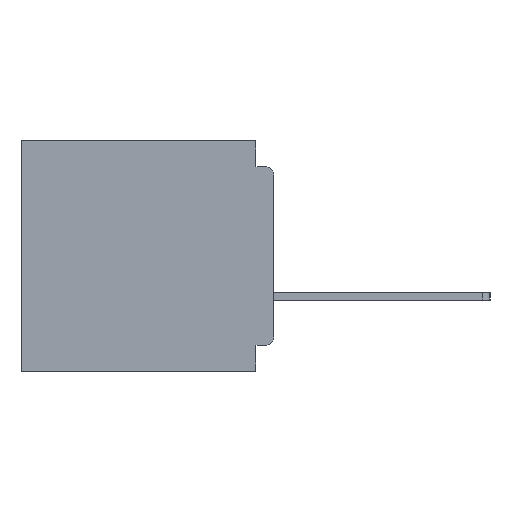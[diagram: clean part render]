
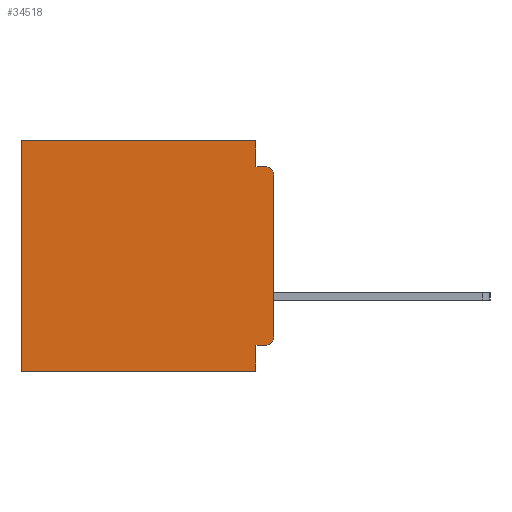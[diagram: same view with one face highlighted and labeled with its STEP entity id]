
A CAD part, left-side view. The second image highlights one B-rep face of the part: STEP entity #34518.
In plain terms, the highlighted planar face has unit normal (-1, 0, 0).
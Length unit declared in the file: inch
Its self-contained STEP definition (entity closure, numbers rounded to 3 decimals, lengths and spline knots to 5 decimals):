
#364 = DIRECTION ( 'NONE',  ( 0., 0., -1. ) ) ;
#880 = VERTEX_POINT ( 'NONE', #19488 ) ;
#1233 = EDGE_CURVE ( 'NONE', #1501, #36022, #8729, .T. ) ;
#1242 = EDGE_CURVE ( 'NONE', #15612, #1501, #24588, .T. ) ;
#1501 = VERTEX_POINT ( 'NONE', #20663 ) ;
#2555 = DIRECTION ( 'NONE',  ( 0., -1., 0. ) ) ;
#2652 = DIRECTION ( 'NONE',  ( -1., 0., 0. ) ) ;
#3565 = VECTOR ( 'NONE', #2555, 39.37008 ) ;
#4012 = LINE ( 'NONE', #10964, #20931 ) ;
#4858 = EDGE_CURVE ( 'NONE', #30091, #30769, #34595, .T. ) ;
#5590 = EDGE_CURVE ( 'NONE', #15612, #20158, #31104, .T. ) ;
#5724 = AXIS2_PLACEMENT_3D ( 'NONE', #21704, #2652, #24870 ) ;
#6927 = CARTESIAN_POINT ( 'NONE',  ( 0.3, 0., -0.4 ) ) ;
#7336 = LINE ( 'NONE', #33890, #24201 ) ;
#7549 = CARTESIAN_POINT ( 'NONE',  ( 0.3, 0., -0.4 ) ) ;
#8361 = ORIENTED_EDGE ( 'NONE', *, *, #8889, .F. ) ;
#8549 = DIRECTION ( 'NONE',  ( -1., 0., 0. ) ) ;
#8682 = AXIS2_PLACEMENT_3D ( 'NONE', #7549, #17140, #39043 ) ;
#8729 = LINE ( 'NONE', #22345, #25586 ) ;
#8889 = EDGE_CURVE ( 'NONE', #20158, #17892, #27850, .T. ) ;
#9455 = VECTOR ( 'NONE', #16141, 39.37008 ) ;
#10663 = VECTOR ( 'NONE', #364, 39.37008 ) ;
#10964 = CARTESIAN_POINT ( 'NONE',  ( 0.3, 0., -0.4 ) ) ;
#12953 = CARTESIAN_POINT ( 'NONE',  ( 0.3, 0.031, -0.4 ) ) ;
#13448 = CARTESIAN_POINT ( 'NONE',  ( 0.3, 0.031, 0. ) ) ;
#13936 = PLANE ( 'NONE',  #8682 ) ;
#14326 = ORIENTED_EDGE ( 'NONE', *, *, #34737, .T. ) ;
#14331 = VECTOR ( 'NONE', #19848, 39.37008 ) ;
#15174 = VECTOR ( 'NONE', #21255, 39.37008 ) ;
#15340 = CARTESIAN_POINT ( 'NONE',  ( 0.3, 0., -0.045 ) ) ;
#15386 = ORIENTED_EDGE ( 'NONE', *, *, #24315, .F. ) ;
#15612 = VERTEX_POINT ( 'NONE', #32898 ) ;
#16141 = DIRECTION ( 'NONE',  ( 0., 0., -1. ) ) ;
#16449 = ORIENTED_EDGE ( 'NONE', *, *, #1233, .T. ) ;
#17140 = DIRECTION ( 'NONE',  ( 1., 0., 0. ) ) ;
#17245 = CARTESIAN_POINT ( 'NONE',  ( 0.3, 0.015, -0.355 ) ) ;
#17627 = CARTESIAN_POINT ( 'NONE',  ( 0.3, 0.031, -0.045 ) ) ;
#17892 = VERTEX_POINT ( 'NONE', #24485 ) ;
#19488 = CARTESIAN_POINT ( 'NONE',  ( 0.3, 0., -0.34 ) ) ;
#19553 = ORIENTED_EDGE ( 'NONE', *, *, #5590, .F. ) ;
#19848 = DIRECTION ( 'NONE',  ( 0., 0., -1. ) ) ;
#20103 = EDGE_CURVE ( 'NONE', #30769, #36022, #4012, .T. ) ;
#20126 = LINE ( 'NONE', #6927, #10663 ) ;
#20158 = VERTEX_POINT ( 'NONE', #17627 ) ;
#20663 = CARTESIAN_POINT ( 'NONE',  ( 0.3, 0.437, 0. ) ) ;
#20697 = CIRCLE ( 'NONE', #5724, 0.015 ) ;
#20931 = VECTOR ( 'NONE', #29861, 39.37008 ) ;
#21123 = DIRECTION ( 'NONE',  ( 0., 0., -1. ) ) ;
#21216 = FACE_OUTER_BOUND ( 'NONE', #29043, .T. ) ;
#21255 = DIRECTION ( 'NONE',  ( 0., 1., 0. ) ) ;
#21395 = CARTESIAN_POINT ( 'NONE',  ( 0.3, 0., 0. ) ) ;
#21704 = CARTESIAN_POINT ( 'NONE',  ( 0.3, 0.015, -0.06 ) ) ;
#22178 = CARTESIAN_POINT ( 'NONE',  ( 0.3, 0.437, -0.4 ) ) ;
#22345 = CARTESIAN_POINT ( 'NONE',  ( 0.3, 0.437, -0.4 ) ) ;
#23362 = EDGE_CURVE ( 'NONE', #25110, #880, #28987, .T. ) ;
#24201 = VECTOR ( 'NONE', #36997, 39.37008 ) ;
#24315 = EDGE_CURVE ( 'NONE', #33473, #880, #20126, .T. ) ;
#24485 = CARTESIAN_POINT ( 'NONE',  ( 0.3, 0.015, -0.045 ) ) ;
#24588 = LINE ( 'NONE', #21395, #15174 ) ;
#24870 = DIRECTION ( 'NONE',  ( 0., 0., -1. ) ) ;
#24985 = CARTESIAN_POINT ( 'NONE',  ( 0.3, 0.031, -0.355 ) ) ;
#25110 = VERTEX_POINT ( 'NONE', #17245 ) ;
#25551 = ORIENTED_EDGE ( 'NONE', *, *, #20103, .F. ) ;
#25586 = VECTOR ( 'NONE', #21123, 39.37008 ) ;
#26497 = EDGE_CURVE ( 'NONE', #25110, #30091, #7336, .T. ) ;
#26961 = AXIS2_PLACEMENT_3D ( 'NONE', #27501, #8549, #30621 ) ;
#27440 = CARTESIAN_POINT ( 'NONE',  ( 0.3, 0., -0.06 ) ) ;
#27501 = CARTESIAN_POINT ( 'NONE',  ( 0.3, 0.015, -0.34 ) ) ;
#27850 = LINE ( 'NONE', #15340, #3565 ) ;
#28987 = CIRCLE ( 'NONE', #26961, 0.015 ) ;
#29043 = EDGE_LOOP ( 'NONE', ( #15386, #14326, #8361, #19553, #30883, #16449, #25551, #31829, #31611, #35173 ) ) ;
#29861 = DIRECTION ( 'NONE',  ( 0., 1., 0. ) ) ;
#30091 = VERTEX_POINT ( 'NONE', #24985 ) ;
#30621 = DIRECTION ( 'NONE',  ( 0., 0., -1. ) ) ;
#30769 = VERTEX_POINT ( 'NONE', #34025 ) ;
#30883 = ORIENTED_EDGE ( 'NONE', *, *, #1242, .T. ) ;
#31104 = LINE ( 'NONE', #13448, #14331 ) ;
#31611 = ORIENTED_EDGE ( 'NONE', *, *, #26497, .F. ) ;
#31829 = ORIENTED_EDGE ( 'NONE', *, *, #4858, .F. ) ;
#32898 = CARTESIAN_POINT ( 'NONE',  ( 0.3, 0.031, 0. ) ) ;
#33473 = VERTEX_POINT ( 'NONE', #27440 ) ;
#33890 = CARTESIAN_POINT ( 'NONE',  ( 0.3, 0., -0.355 ) ) ;
#34025 = CARTESIAN_POINT ( 'NONE',  ( 0.3, 0.031, -0.4 ) ) ;
#34518 = ADVANCED_FACE ( 'NONE', ( #21216 ), #13936, .F. ) ;
#34595 = LINE ( 'NONE', #12953, #9455 ) ;
#34737 = EDGE_CURVE ( 'NONE', #33473, #17892, #20697, .T. ) ;
#35173 = ORIENTED_EDGE ( 'NONE', *, *, #23362, .T. ) ;
#36022 = VERTEX_POINT ( 'NONE', #22178 ) ;
#36997 = DIRECTION ( 'NONE',  ( 0., 1., 0. ) ) ;
#39043 = DIRECTION ( 'NONE',  ( 0., 0., -1. ) ) ;
